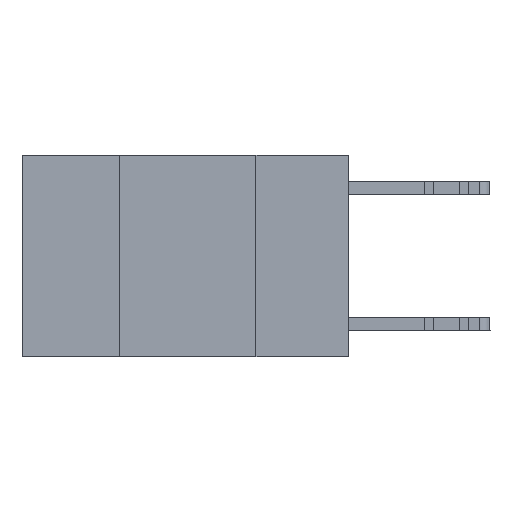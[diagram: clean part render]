
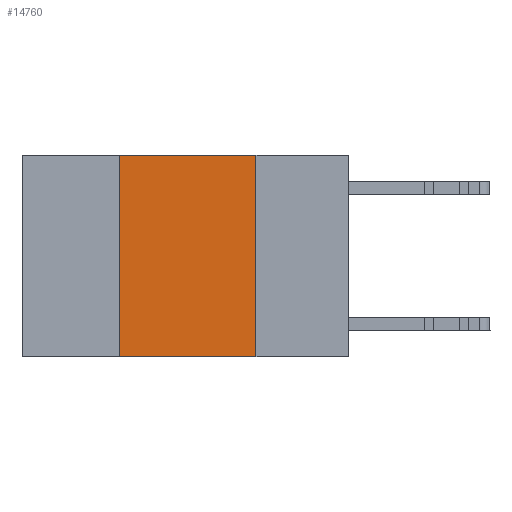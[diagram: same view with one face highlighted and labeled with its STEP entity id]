
A CAD part, left-side view. The second image highlights one B-rep face of the part: STEP entity #14760.
In plain terms, the highlighted planar face has unit normal (-1, 0, 0).
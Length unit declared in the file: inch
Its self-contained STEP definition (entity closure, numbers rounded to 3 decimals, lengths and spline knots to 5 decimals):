
#349 = CARTESIAN_POINT ( 'NONE',  ( 0., 0.6, 0. ) ) ;
#556 = DIRECTION ( 'NONE',  ( 0., -1., 0. ) ) ;
#666 = DIRECTION ( 'NONE',  ( 0., 0., -1. ) ) ;
#1077 = DIRECTION ( 'NONE',  ( 0., 0., -1. ) ) ;
#2221 = EDGE_CURVE ( 'NONE', #13678, #8623, #15515, .T. ) ;
#2570 = ORIENTED_EDGE ( 'NONE', *, *, #22285, .T. ) ;
#3123 = VECTOR ( 'NONE', #1077, 39.37008 ) ;
#3337 = FACE_OUTER_BOUND ( 'NONE', #6391, .T. ) ;
#5065 = LINE ( 'NONE', #8032, #12072 ) ;
#5825 = AXIS2_PLACEMENT_3D ( 'NONE', #349, #23439, #666 ) ;
#6391 = EDGE_LOOP ( 'NONE', ( #28997, #31393, #29207, #2570 ) ) ;
#8032 = CARTESIAN_POINT ( 'NONE',  ( 0., 0.6, 0. ) ) ;
#8057 = CARTESIAN_POINT ( 'NONE',  ( 0., 0.17, 0. ) ) ;
#8623 = VERTEX_POINT ( 'NONE', #26330 ) ;
#12072 = VECTOR ( 'NONE', #15206, 39.37008 ) ;
#12091 = EDGE_CURVE ( 'NONE', #8623, #13190, #5065, .T. ) ;
#13029 = DIRECTION ( 'NONE',  ( 0., 0., 1. ) ) ;
#13190 = VERTEX_POINT ( 'NONE', #29863 ) ;
#13678 = VERTEX_POINT ( 'NONE', #19069 ) ;
#13846 = EDGE_CURVE ( 'NONE', #13190, #29948, #23689, .T. ) ;
#14639 = VECTOR ( 'NONE', #13029, 39.37008 ) ;
#14760 = ADVANCED_FACE ( 'NONE', ( #3337 ), #23284, .F. ) ;
#15206 = DIRECTION ( 'NONE',  ( 0., -1., 0. ) ) ;
#15515 = LINE ( 'NONE', #23000, #14639 ) ;
#19069 = CARTESIAN_POINT ( 'NONE',  ( 0., 0.42, -0.37 ) ) ;
#19123 = VECTOR ( 'NONE', #556, 39.37008 ) ;
#22285 = EDGE_CURVE ( 'NONE', #13678, #29948, #23179, .T. ) ;
#23000 = CARTESIAN_POINT ( 'NONE',  ( 0., 0.42, 0. ) ) ;
#23179 = LINE ( 'NONE', #28661, #19123 ) ;
#23284 = PLANE ( 'NONE',  #5825 ) ;
#23439 = DIRECTION ( 'NONE',  ( 1., 0., 0. ) ) ;
#23689 = LINE ( 'NONE', #8057, #3123 ) ;
#24503 = CARTESIAN_POINT ( 'NONE',  ( 0., 0.17, -0.37 ) ) ;
#26330 = CARTESIAN_POINT ( 'NONE',  ( 0., 0.42, 0. ) ) ;
#28661 = CARTESIAN_POINT ( 'NONE',  ( 0., 0.6, -0.37 ) ) ;
#28997 = ORIENTED_EDGE ( 'NONE', *, *, #13846, .F. ) ;
#29207 = ORIENTED_EDGE ( 'NONE', *, *, #2221, .F. ) ;
#29863 = CARTESIAN_POINT ( 'NONE',  ( 0., 0.17, 0. ) ) ;
#29948 = VERTEX_POINT ( 'NONE', #24503 ) ;
#31393 = ORIENTED_EDGE ( 'NONE', *, *, #12091, .F. ) ;
